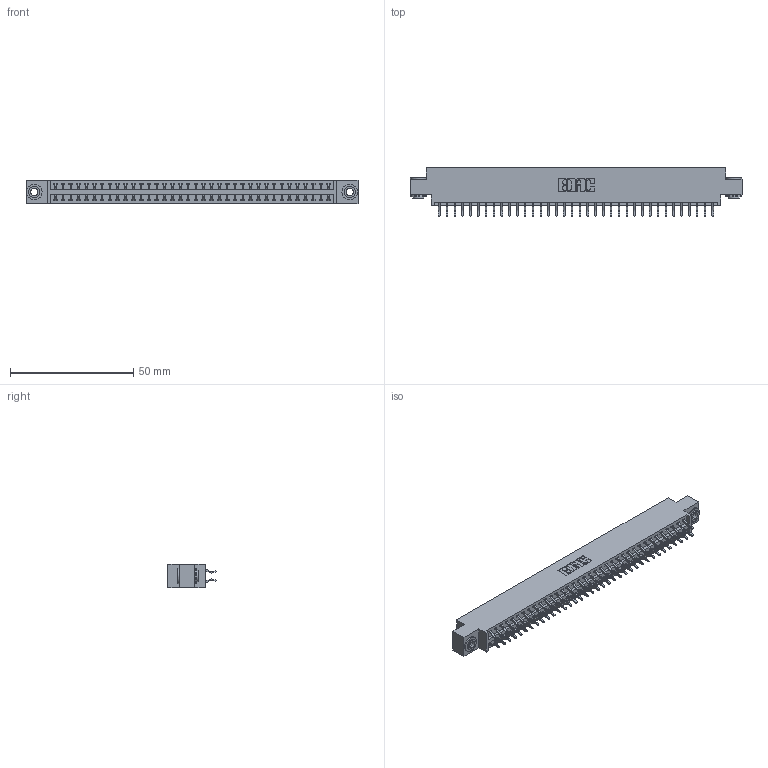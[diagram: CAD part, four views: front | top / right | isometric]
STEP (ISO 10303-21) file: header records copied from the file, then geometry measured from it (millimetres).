
FILE_DESCRIPTION (( 'STEP AP203' ), '1' );
FILE_NAME ('346-072-556-803.STEP', '2022-05-25T00:37:55', ( '' ), ( '' ), 'SwSTEP 2.0', 'SolidWorks 2020', '' );
FILE_SCHEMA (( 'CONFIG_CONTROL_DESIGN' ));
Length unit declared in the file: inch
Products named in the file (4): 346 Part_0.170 Offset - 0.156 Dia-TH; 345-250-002_345-250-002-102; 346-072-556-803; 345-292-001_556 Tail
Assembly tree (75 placements, depth 2):
  346-072-556-803
    346 Part_0.170 Offset - 0.156 Dia-TH
    345-292-001_556 Tail  x72
    345-250-002_345-250-002-102  x2
Bounding box: 134.87 x 19.57 x 9.4 mm (x, y, z)
Volume: 12949.1 mm3; surface area: 18066.6 mm2
Topology: 75 solids, 75 shells, 4354 faces, 12909 edges, 8506 vertices
Faces by surface type: plane 2912, cylinder 1434, cone 8
Entity records: 25720 total; most frequent: CARTESIAN_POINT 4245, ORIENTED_EDGE 4158, DIRECTION 3809, EDGE_CURVE 2079, LINE 1771, VECTOR 1771, VERTEX_POINT 1382, AXIS2_PLACEMENT_3D 1019
